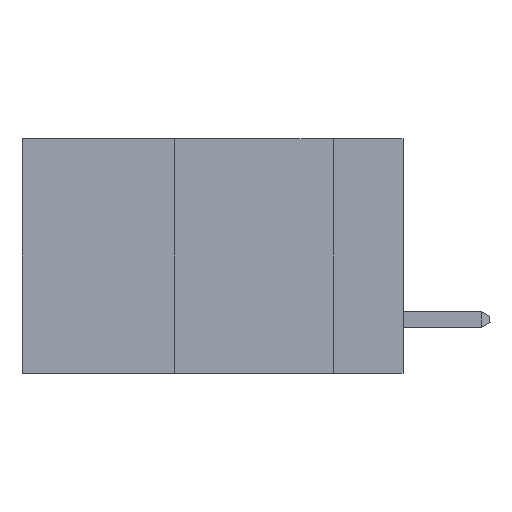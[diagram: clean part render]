
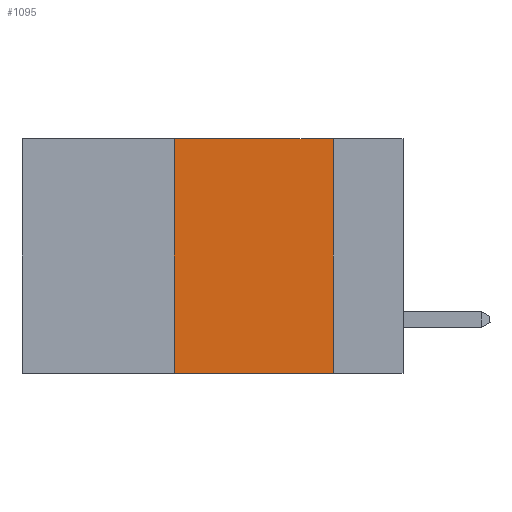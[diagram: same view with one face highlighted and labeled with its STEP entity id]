
A CAD part, left-side view. The second image highlights one B-rep face of the part: STEP entity #1095.
In plain terms, the highlighted planar face has unit normal (-1, 0, 0).
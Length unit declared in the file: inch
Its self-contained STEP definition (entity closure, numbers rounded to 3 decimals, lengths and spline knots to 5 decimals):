
#133 = EDGE_CURVE ( 'NONE', #1053, #19501, #3131, .T. ) ;
#183 = VECTOR ( 'NONE', #1479, 39.37008 ) ;
#574 = EDGE_LOOP ( 'NONE', ( #12470, #17739, #11001, #14564 ) ) ;
#728 = DIRECTION ( 'NONE',  ( 0., 0., -1. ) ) ;
#738 = DIRECTION ( 'NONE',  ( 0., 0., 1. ) ) ;
#994 = FACE_OUTER_BOUND ( 'NONE', #574, .T. ) ;
#1053 = VERTEX_POINT ( 'NONE', #20667 ) ;
#1073 = VERTEX_POINT ( 'NONE', #13681 ) ;
#1095 = ADVANCED_FACE ( 'NONE', ( #994 ), #9292, .F. ) ;
#1479 = DIRECTION ( 'NONE',  ( 0., 0., -1. ) ) ;
#1764 = LINE ( 'NONE', #3414, #183 ) ;
#1893 = VECTOR ( 'NONE', #10290, 39.37008 ) ;
#2558 = DIRECTION ( 'NONE',  ( 0., -1., 0. ) ) ;
#3131 = LINE ( 'NONE', #5853, #9218 ) ;
#3414 = CARTESIAN_POINT ( 'NONE',  ( 0., 0.11, 0. ) ) ;
#4062 = CARTESIAN_POINT ( 'NONE',  ( 0., 0.6, 0. ) ) ;
#5853 = CARTESIAN_POINT ( 'NONE',  ( 0., 0.6, 0. ) ) ;
#7473 = DIRECTION ( 'NONE',  ( 1., 0., 0. ) ) ;
#7984 = LINE ( 'NONE', #17001, #1893 ) ;
#8519 = EDGE_CURVE ( 'NONE', #19501, #14773, #1764, .T. ) ;
#9218 = VECTOR ( 'NONE', #2558, 39.37008 ) ;
#9292 = PLANE ( 'NONE',  #13593 ) ;
#9524 = CARTESIAN_POINT ( 'NONE',  ( 0., 0.36, 0. ) ) ;
#10290 = DIRECTION ( 'NONE',  ( 0., -1., 0. ) ) ;
#11001 = ORIENTED_EDGE ( 'NONE', *, *, #16640, .F. ) ;
#11041 = EDGE_CURVE ( 'NONE', #1073, #14773, #7984, .T. ) ;
#12232 = LINE ( 'NONE', #9524, #18571 ) ;
#12470 = ORIENTED_EDGE ( 'NONE', *, *, #8519, .F. ) ;
#13593 = AXIS2_PLACEMENT_3D ( 'NONE', #4062, #7473, #728 ) ;
#13681 = CARTESIAN_POINT ( 'NONE',  ( 0., 0.36, -0.37 ) ) ;
#13863 = CARTESIAN_POINT ( 'NONE',  ( 0., 0.11, -0.37 ) ) ;
#14297 = CARTESIAN_POINT ( 'NONE',  ( 0., 0.11, 0. ) ) ;
#14564 = ORIENTED_EDGE ( 'NONE', *, *, #11041, .T. ) ;
#14773 = VERTEX_POINT ( 'NONE', #13863 ) ;
#16640 = EDGE_CURVE ( 'NONE', #1073, #1053, #12232, .T. ) ;
#17001 = CARTESIAN_POINT ( 'NONE',  ( 0., 0.6, -0.37 ) ) ;
#17739 = ORIENTED_EDGE ( 'NONE', *, *, #133, .F. ) ;
#18571 = VECTOR ( 'NONE', #738, 39.37008 ) ;
#19501 = VERTEX_POINT ( 'NONE', #14297 ) ;
#20667 = CARTESIAN_POINT ( 'NONE',  ( 0., 0.36, 0. ) ) ;
